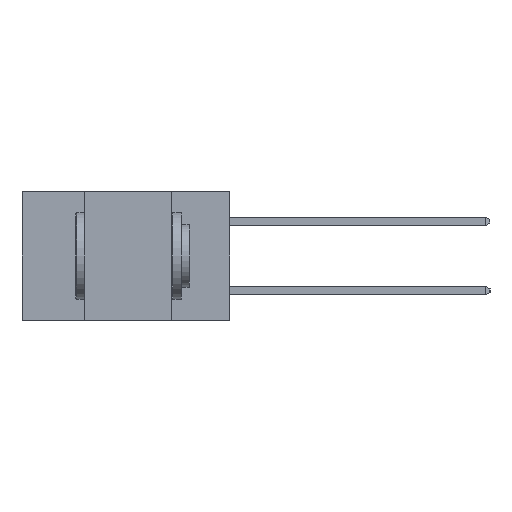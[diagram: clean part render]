
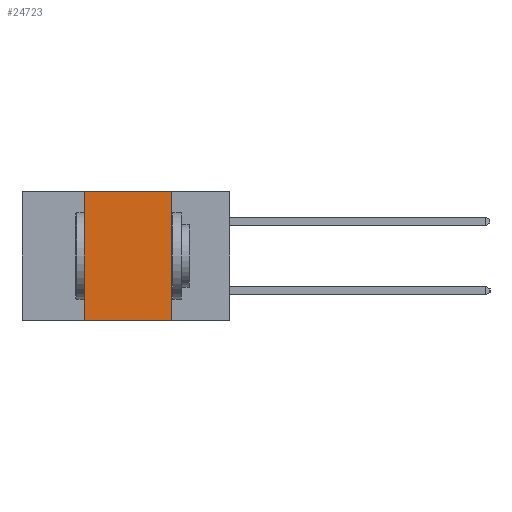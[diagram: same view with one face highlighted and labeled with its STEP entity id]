
A CAD part, left-side view. The second image highlights one B-rep face of the part: STEP entity #24723.
In plain terms, the highlighted planar face has unit normal (-1, 0, 0).
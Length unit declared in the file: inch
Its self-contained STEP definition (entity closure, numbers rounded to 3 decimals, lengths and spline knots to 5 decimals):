
#1073 = VECTOR ( 'NONE', #7725, 39.37008 ) ;
#1942 = DIRECTION ( 'NONE',  ( 0., -1., 0. ) ) ;
#2780 = ORIENTED_EDGE ( 'NONE', *, *, #16916, .F. ) ;
#3076 = VERTEX_POINT ( 'NONE', #3134 ) ;
#3134 = CARTESIAN_POINT ( 'NONE',  ( 0., 0.42, 0. ) ) ;
#4045 = DIRECTION ( 'NONE',  ( 0., 0., 1. ) ) ;
#4057 = LINE ( 'NONE', #18289, #14283 ) ;
#4541 = PLANE ( 'NONE',  #7779 ) ;
#5661 = CARTESIAN_POINT ( 'NONE',  ( 0., 0.6, 0. ) ) ;
#5988 = FACE_OUTER_BOUND ( 'NONE', #24238, .T. ) ;
#6602 = CARTESIAN_POINT ( 'NONE',  ( 0., 0.6, 0. ) ) ;
#7460 = CARTESIAN_POINT ( 'NONE',  ( 0., 0.17, -0.37 ) ) ;
#7725 = DIRECTION ( 'NONE',  ( 0., -1., 0. ) ) ;
#7779 = AXIS2_PLACEMENT_3D ( 'NONE', #6602, #8670, #22804 ) ;
#7963 = LINE ( 'NONE', #16296, #23447 ) ;
#8336 = EDGE_CURVE ( 'NONE', #18816, #21506, #7963, .T. ) ;
#8670 = DIRECTION ( 'NONE',  ( 1., 0., 0. ) ) ;
#10946 = EDGE_CURVE ( 'NONE', #3076, #15786, #17427, .T. ) ;
#13619 = DIRECTION ( 'NONE',  ( 0., 0., -1. ) ) ;
#14283 = VECTOR ( 'NONE', #4045, 39.37008 ) ;
#15271 = ORIENTED_EDGE ( 'NONE', *, *, #8336, .T. ) ;
#15786 = VERTEX_POINT ( 'NONE', #17041 ) ;
#15894 = ORIENTED_EDGE ( 'NONE', *, *, #23087, .F. ) ;
#16296 = CARTESIAN_POINT ( 'NONE',  ( 0., 0.6, -0.37 ) ) ;
#16916 = EDGE_CURVE ( 'NONE', #18816, #3076, #4057, .T. ) ;
#17041 = CARTESIAN_POINT ( 'NONE',  ( 0., 0.17, 0. ) ) ;
#17427 = LINE ( 'NONE', #5661, #1073 ) ;
#18289 = CARTESIAN_POINT ( 'NONE',  ( 0., 0.42, -0.37 ) ) ;
#18741 = CARTESIAN_POINT ( 'NONE',  ( 0., 0.17, -0.37 ) ) ;
#18816 = VERTEX_POINT ( 'NONE', #24530 ) ;
#19130 = VECTOR ( 'NONE', #13619, 39.37008 ) ;
#21506 = VERTEX_POINT ( 'NONE', #18741 ) ;
#22804 = DIRECTION ( 'NONE',  ( 0., 0., -1. ) ) ;
#23087 = EDGE_CURVE ( 'NONE', #15786, #21506, #25051, .T. ) ;
#23447 = VECTOR ( 'NONE', #1942, 39.37008 ) ;
#23695 = ORIENTED_EDGE ( 'NONE', *, *, #10946, .F. ) ;
#24238 = EDGE_LOOP ( 'NONE', ( #15894, #23695, #2780, #15271 ) ) ;
#24530 = CARTESIAN_POINT ( 'NONE',  ( 0., 0.42, -0.37 ) ) ;
#24723 = ADVANCED_FACE ( 'NONE', ( #5988 ), #4541, .F. ) ;
#25051 = LINE ( 'NONE', #7460, #19130 ) ;
